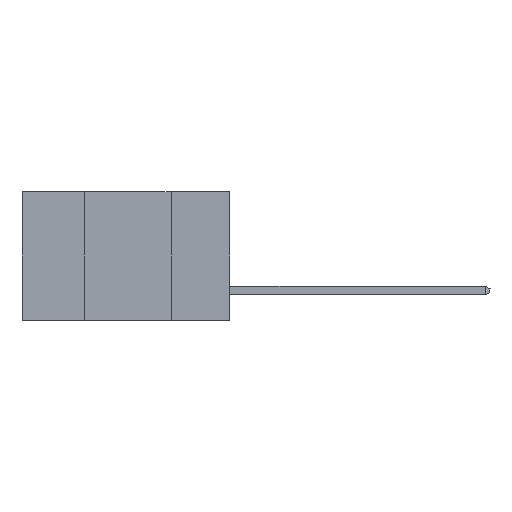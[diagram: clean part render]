
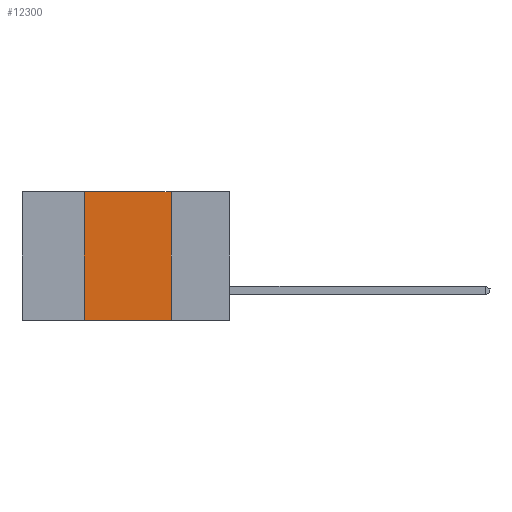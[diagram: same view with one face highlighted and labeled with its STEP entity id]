
A CAD part, left-side view. The second image highlights one B-rep face of the part: STEP entity #12300.
In plain terms, the highlighted planar face has unit normal (-1, 0, 0).
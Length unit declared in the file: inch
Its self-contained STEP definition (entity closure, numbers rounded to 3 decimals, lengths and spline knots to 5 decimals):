
#30 = VERTEX_POINT ( 'NONE', #829 ) ;
#738 = FACE_OUTER_BOUND ( 'NONE', #16551, .T. ) ;
#829 = CARTESIAN_POINT ( 'NONE',  ( 0., 0.17, -0.37 ) ) ;
#1189 = ORIENTED_EDGE ( 'NONE', *, *, #5105, .F. ) ;
#2109 = VECTOR ( 'NONE', #16851, 39.37008 ) ;
#3165 = ORIENTED_EDGE ( 'NONE', *, *, #11569, .F. ) ;
#3301 = ORIENTED_EDGE ( 'NONE', *, *, #4282, .F. ) ;
#3816 = ORIENTED_EDGE ( 'NONE', *, *, #7915, .T. ) ;
#4282 = EDGE_CURVE ( 'NONE', #14853, #30, #9110, .T. ) ;
#4729 = LINE ( 'NONE', #11046, #12940 ) ;
#4878 = CARTESIAN_POINT ( 'NONE',  ( 0., 0.6, -0.37 ) ) ;
#5105 = EDGE_CURVE ( 'NONE', #14899, #14853, #5826, .T. ) ;
#5110 = PLANE ( 'NONE',  #12289 ) ;
#5209 = DIRECTION ( 'NONE',  ( 0., -1., 0. ) ) ;
#5224 = DIRECTION ( 'NONE',  ( 0., 0., -1. ) ) ;
#5574 = VERTEX_POINT ( 'NONE', #13588 ) ;
#5826 = LINE ( 'NONE', #16833, #15647 ) ;
#6134 = VECTOR ( 'NONE', #11750, 39.37008 ) ;
#6544 = LINE ( 'NONE', #4878, #6134 ) ;
#7915 = EDGE_CURVE ( 'NONE', #5574, #30, #6544, .T. ) ;
#8365 = DIRECTION ( 'NONE',  ( 0., 0., 1. ) ) ;
#9110 = LINE ( 'NONE', #10356, #2109 ) ;
#10356 = CARTESIAN_POINT ( 'NONE',  ( 0., 0.17, 0. ) ) ;
#11046 = CARTESIAN_POINT ( 'NONE',  ( 0., 0.42, 0. ) ) ;
#11569 = EDGE_CURVE ( 'NONE', #5574, #14899, #4729, .T. ) ;
#11750 = DIRECTION ( 'NONE',  ( 0., -1., 0. ) ) ;
#12289 = AXIS2_PLACEMENT_3D ( 'NONE', #15694, #16845, #5224 ) ;
#12300 = ADVANCED_FACE ( 'NONE', ( #738 ), #5110, .F. ) ;
#12940 = VECTOR ( 'NONE', #8365, 39.37008 ) ;
#13588 = CARTESIAN_POINT ( 'NONE',  ( 0., 0.42, -0.37 ) ) ;
#14500 = CARTESIAN_POINT ( 'NONE',  ( 0., 0.42, 0. ) ) ;
#14853 = VERTEX_POINT ( 'NONE', #15623 ) ;
#14899 = VERTEX_POINT ( 'NONE', #14500 ) ;
#15623 = CARTESIAN_POINT ( 'NONE',  ( 0., 0.17, 0. ) ) ;
#15647 = VECTOR ( 'NONE', #5209, 39.37008 ) ;
#15694 = CARTESIAN_POINT ( 'NONE',  ( 0., 0.6, 0. ) ) ;
#16551 = EDGE_LOOP ( 'NONE', ( #3301, #1189, #3165, #3816 ) ) ;
#16833 = CARTESIAN_POINT ( 'NONE',  ( 0., 0.6, 0. ) ) ;
#16845 = DIRECTION ( 'NONE',  ( 1., 0., 0. ) ) ;
#16851 = DIRECTION ( 'NONE',  ( 0., 0., -1. ) ) ;
